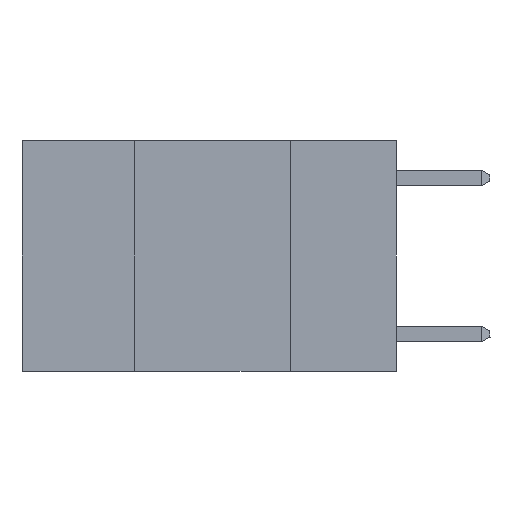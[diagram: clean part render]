
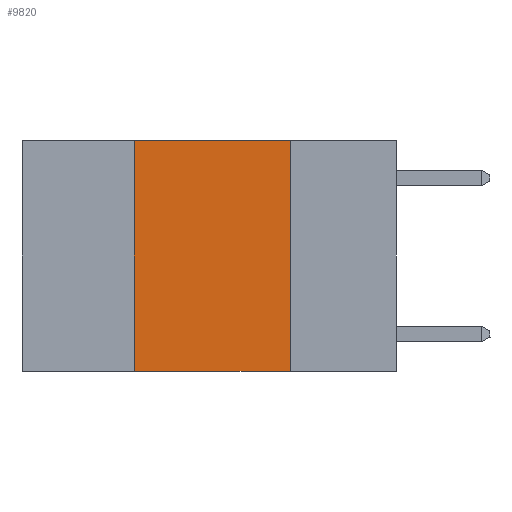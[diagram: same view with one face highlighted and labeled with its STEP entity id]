
A CAD part, left-side view. The second image highlights one B-rep face of the part: STEP entity #9820.
In plain terms, the highlighted planar face has unit normal (-1, 0, 0).
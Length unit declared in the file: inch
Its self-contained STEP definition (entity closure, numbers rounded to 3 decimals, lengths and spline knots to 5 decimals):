
#337 = DIRECTION ( 'NONE',  ( 0., -1., 0. ) ) ;
#1618 = CARTESIAN_POINT ( 'NONE',  ( 0., 0.17, 0. ) ) ;
#1986 = CARTESIAN_POINT ( 'NONE',  ( 0., 0.6, 0. ) ) ;
#2655 = EDGE_CURVE ( 'NONE', #4562, #3380, #5239, .T. ) ;
#3114 = CARTESIAN_POINT ( 'NONE',  ( 0., 0.42, -0.37 ) ) ;
#3380 = VERTEX_POINT ( 'NONE', #6218 ) ;
#4263 = ORIENTED_EDGE ( 'NONE', *, *, #8280, .T. ) ;
#4562 = VERTEX_POINT ( 'NONE', #3114 ) ;
#5068 = EDGE_CURVE ( 'NONE', #5773, #5387, #14970, .T. ) ;
#5129 = CARTESIAN_POINT ( 'NONE',  ( 0., 0.17, 0. ) ) ;
#5239 = LINE ( 'NONE', #9022, #8414 ) ;
#5343 = ORIENTED_EDGE ( 'NONE', *, *, #5068, .F. ) ;
#5387 = VERTEX_POINT ( 'NONE', #10770 ) ;
#5760 = ORIENTED_EDGE ( 'NONE', *, *, #11343, .F. ) ;
#5773 = VERTEX_POINT ( 'NONE', #5129 ) ;
#6218 = CARTESIAN_POINT ( 'NONE',  ( 0., 0.42, 0. ) ) ;
#6254 = VECTOR ( 'NONE', #337, 39.37008 ) ;
#6987 = LINE ( 'NONE', #12361, #6254 ) ;
#7535 = EDGE_LOOP ( 'NONE', ( #5343, #5760, #11446, #4263 ) ) ;
#7699 = DIRECTION ( 'NONE',  ( 0., 0., 1. ) ) ;
#8280 = EDGE_CURVE ( 'NONE', #4562, #5387, #6987, .T. ) ;
#8414 = VECTOR ( 'NONE', #7699, 39.37008 ) ;
#8656 = VECTOR ( 'NONE', #10973, 39.37008 ) ;
#9022 = CARTESIAN_POINT ( 'NONE',  ( 0., 0.42, 0. ) ) ;
#9338 = CARTESIAN_POINT ( 'NONE',  ( 0., 0.6, 0. ) ) ;
#9820 = ADVANCED_FACE ( 'NONE', ( #13928 ), #9949, .F. ) ;
#9851 = VECTOR ( 'NONE', #11863, 39.37008 ) ;
#9949 = PLANE ( 'NONE',  #15016 ) ;
#10770 = CARTESIAN_POINT ( 'NONE',  ( 0., 0.17, -0.37 ) ) ;
#10973 = DIRECTION ( 'NONE',  ( 0., 0., -1. ) ) ;
#11343 = EDGE_CURVE ( 'NONE', #3380, #5773, #15853, .T. ) ;
#11429 = DIRECTION ( 'NONE',  ( 0., 0., -1. ) ) ;
#11446 = ORIENTED_EDGE ( 'NONE', *, *, #2655, .F. ) ;
#11516 = DIRECTION ( 'NONE',  ( 1., 0., 0. ) ) ;
#11863 = DIRECTION ( 'NONE',  ( 0., -1., 0. ) ) ;
#12361 = CARTESIAN_POINT ( 'NONE',  ( 0., 0.6, -0.37 ) ) ;
#13928 = FACE_OUTER_BOUND ( 'NONE', #7535, .T. ) ;
#14970 = LINE ( 'NONE', #1618, #8656 ) ;
#15016 = AXIS2_PLACEMENT_3D ( 'NONE', #1986, #11516, #11429 ) ;
#15853 = LINE ( 'NONE', #9338, #9851 ) ;
